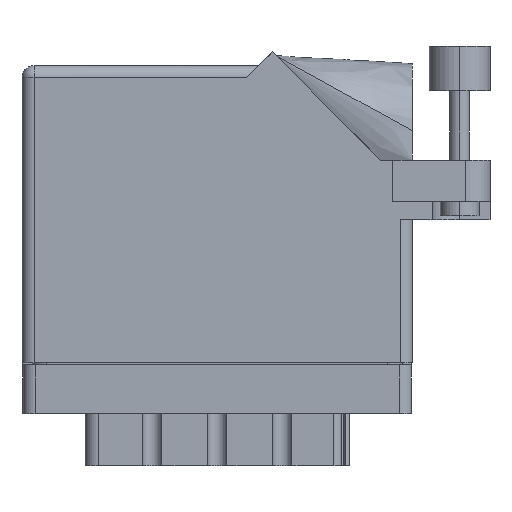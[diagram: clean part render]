
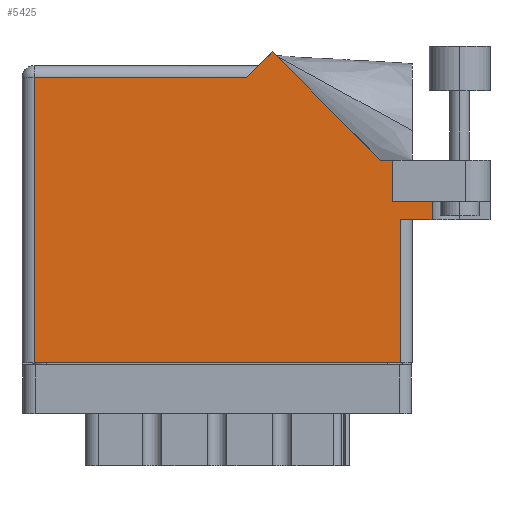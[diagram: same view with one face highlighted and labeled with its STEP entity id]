
A CAD part, front view. The second image highlights one B-rep face of the part: STEP entity #5425.
In plain terms, the highlighted face is planar.
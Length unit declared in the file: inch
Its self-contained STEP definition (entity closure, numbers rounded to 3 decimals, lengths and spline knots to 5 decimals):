
#279 = EDGE_CURVE ( 'NONE', #6569, #7524, #4848, .T. ) ;
#532 = LINE ( 'NONE', #20864, #30896 ) ;
#762 = LINE ( 'NONE', #24000, #18987 ) ;
#1040 = DIRECTION ( 'NONE',  ( 0., 1., 0. ) ) ;
#1169 = DIRECTION ( 'NONE',  ( 1., 0., 0. ) ) ;
#1285 = VECTOR ( 'NONE', #21340, 39.37008 ) ;
#1596 = LINE ( 'NONE', #26831, #20621 ) ;
#1717 = EDGE_CURVE ( 'NONE', #32760, #32485, #11291, .T. ) ;
#1984 = VECTOR ( 'NONE', #24626, 39.37008 ) ;
#2338 = VECTOR ( 'NONE', #8463, 39.37008 ) ;
#3233 = VECTOR ( 'NONE', #9349, 39.37008 ) ;
#3659 = VERTEX_POINT ( 'NONE', #28725 ) ;
#4147 = ORIENTED_EDGE ( 'NONE', *, *, #23921, .T. ) ;
#4848 = LINE ( 'NONE', #31134, #16184 ) ;
#5110 = ORIENTED_EDGE ( 'NONE', *, *, #26131, .T. ) ;
#5425 = ADVANCED_FACE ( 'NONE', ( #15493 ), #22235, .F. ) ;
#6569 = VERTEX_POINT ( 'NONE', #20222 ) ;
#6713 = CARTESIAN_POINT ( 'NONE',  ( 0., 1.53, 0. ) ) ;
#6724 = CARTESIAN_POINT ( 'NONE',  ( 2.01, 0.737, 0. ) ) ;
#7233 = ORIENTED_EDGE ( 'NONE', *, *, #16714, .T. ) ;
#7524 = VERTEX_POINT ( 'NONE', #20444 ) ;
#7661 = DIRECTION ( 'NONE',  ( 0., -1., 0. ) ) ;
#7669 = VERTEX_POINT ( 'NONE', #28790 ) ;
#7743 = EDGE_CURVE ( 'NONE', #6569, #31011, #1596, .T. ) ;
#8104 = VECTOR ( 'NONE', #7661, 39.37008 ) ;
#8463 = DIRECTION ( 'NONE',  ( -0.707, -0.707, 0. ) ) ;
#8609 = CARTESIAN_POINT ( 'NONE',  ( 1.155, 1.468, 0. ) ) ;
#8707 = VERTEX_POINT ( 'NONE', #22723 ) ;
#8991 = DIRECTION ( 'NONE',  ( 0., -1., 0. ) ) ;
#9339 = CARTESIAN_POINT ( 'NONE',  ( 0.062, 0., 0. ) ) ;
#9349 = DIRECTION ( 'NONE',  ( 1., 0., 0. ) ) ;
#11034 = CARTESIAN_POINT ( 'NONE',  ( 2.41, 1.044, 0. ) ) ;
#11291 = LINE ( 'NONE', #16692, #1984 ) ;
#11408 = LINE ( 'NONE', #11034, #1285 ) ;
#11658 = VERTEX_POINT ( 'NONE', #19946 ) ;
#12198 = VERTEX_POINT ( 'NONE', #12980 ) ;
#12271 = EDGE_CURVE ( 'NONE', #31011, #8707, #14992, .T. ) ;
#12535 = EDGE_CURVE ( 'NONE', #32485, #11658, #29617, .T. ) ;
#12700 = VECTOR ( 'NONE', #28204, 39.37008 ) ;
#12980 = CARTESIAN_POINT ( 'NONE',  ( 1.84442, 1.044, 0. ) ) ;
#13110 = ORIENTED_EDGE ( 'NONE', *, *, #26031, .T. ) ;
#13919 = LINE ( 'NONE', #27885, #12700 ) ;
#13937 = VERTEX_POINT ( 'NONE', #26216 ) ;
#14594 = ORIENTED_EDGE ( 'NONE', *, *, #7743, .F. ) ;
#14992 = LINE ( 'NONE', #28359, #8104 ) ;
#15423 = DIRECTION ( 'NONE',  ( -1., 0., 0. ) ) ;
#15493 = FACE_OUTER_BOUND ( 'NONE', #20105, .T. ) ;
#16184 = VECTOR ( 'NONE', #28858, 39.37008 ) ;
#16692 = CARTESIAN_POINT ( 'NONE',  ( 0., 1.468, 0. ) ) ;
#16714 = EDGE_CURVE ( 'NONE', #7524, #12198, #11408, .T. ) ;
#16980 = ORIENTED_EDGE ( 'NONE', *, *, #21542, .T. ) ;
#18564 = ORIENTED_EDGE ( 'NONE', *, *, #12535, .T. ) ;
#18563 = CARTESIAN_POINT ( 'NONE',  ( 2.1115, 0.831, 0. ) ) ;
#18758 = ORIENTED_EDGE ( 'NONE', *, *, #1717, .T. ) ;
#18987 = VECTOR ( 'NONE', #31616, 39.37008 ) ;
#19946 = CARTESIAN_POINT ( 'NONE',  ( 0.062, 0., 0. ) ) ;
#20105 = EDGE_LOOP ( 'NONE', ( #16980, #4147, #13110, #27213, #14594, #24291, #7233, #5110, #26908, #18758, #18564 ) ) ;
#20222 = CARTESIAN_POINT ( 'NONE',  ( 1.91, 0.831, 0. ) ) ;
#20444 = CARTESIAN_POINT ( 'NONE',  ( 1.91, 1.044, 0. ) ) ;
#20621 = VECTOR ( 'NONE', #1169, 39.37008 ) ;
#20864 = CARTESIAN_POINT ( 'NONE',  ( 1.948, 0.737, 0. ) ) ;
#21340 = DIRECTION ( 'NONE',  ( -1., 0., 0. ) ) ;
#21542 = EDGE_CURVE ( 'NONE', #11658, #13937, #13919, .T. ) ;
#22235 = PLANE ( 'NONE',  #23390 ) ;
#22723 = CARTESIAN_POINT ( 'NONE',  ( 2.1115, 0.737, 0. ) ) ;
#23390 = AXIS2_PLACEMENT_3D ( 'NONE', #6713, #32898, #15423 ) ;
#23921 = EDGE_CURVE ( 'NONE', #13937, #7669, #532, .T. ) ;
#23976 = CARTESIAN_POINT ( 'NONE',  ( 1.217, 1.53, 0. ) ) ;
#24000 = CARTESIAN_POINT ( 'NONE',  ( 1.84442, 1.044, 0. ) ) ;
#24291 = ORIENTED_EDGE ( 'NONE', *, *, #279, .T. ) ;
#24626 = DIRECTION ( 'NONE',  ( -1., 0., 0. ) ) ;
#24768 = VECTOR ( 'NONE', #8991, 39.37008 ) ;
#26031 = EDGE_CURVE ( 'NONE', #7669, #8707, #29529, .T. ) ;
#26131 = EDGE_CURVE ( 'NONE', #12198, #3659, #762, .T. ) ;
#26216 = CARTESIAN_POINT ( 'NONE',  ( 1.948, 0., 0. ) ) ;
#26831 = CARTESIAN_POINT ( 'NONE',  ( 1.91, 0.831, 0. ) ) ;
#26908 = ORIENTED_EDGE ( 'NONE', *, *, #30912, .T. ) ;
#27213 = ORIENTED_EDGE ( 'NONE', *, *, #12271, .F. ) ;
#27885 = CARTESIAN_POINT ( 'NONE',  ( 0., 0., 0. ) ) ;
#28204 = DIRECTION ( 'NONE',  ( 1., 0., 0. ) ) ;
#28359 = CARTESIAN_POINT ( 'NONE',  ( 2.1115, 1.16177, 0. ) ) ;
#28725 = CARTESIAN_POINT ( 'NONE',  ( 1.28771, 1.60071, 0. ) ) ;
#28790 = CARTESIAN_POINT ( 'NONE',  ( 1.948, 0.737, 0. ) ) ;
#28858 = DIRECTION ( 'NONE',  ( 0., 1., 0. ) ) ;
#29529 = LINE ( 'NONE', #6724, #3233 ) ;
#29617 = LINE ( 'NONE', #9339, #24768 ) ;
#30835 = CARTESIAN_POINT ( 'NONE',  ( 0.062, 1.468, 0. ) ) ;
#30896 = VECTOR ( 'NONE', #1040, 39.37008 ) ;
#30912 = EDGE_CURVE ( 'NONE', #3659, #32760, #32314, .T. ) ;
#31011 = VERTEX_POINT ( 'NONE', #18563 ) ;
#31134 = CARTESIAN_POINT ( 'NONE',  ( 1.91, 0.831, 0. ) ) ;
#31616 = DIRECTION ( 'NONE',  ( -0.707, 0.707, 0. ) ) ;
#32314 = LINE ( 'NONE', #23976, #2338 ) ;
#32485 = VERTEX_POINT ( 'NONE', #30835 ) ;
#32760 = VERTEX_POINT ( 'NONE', #8609 ) ;
#32898 = DIRECTION ( 'NONE',  ( 0., 0., -1. ) ) ;
